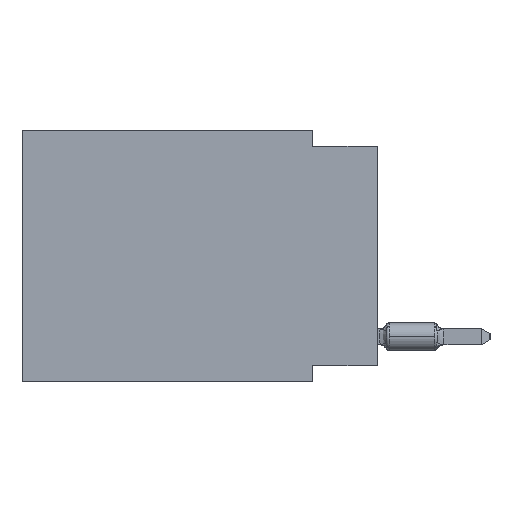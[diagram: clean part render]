
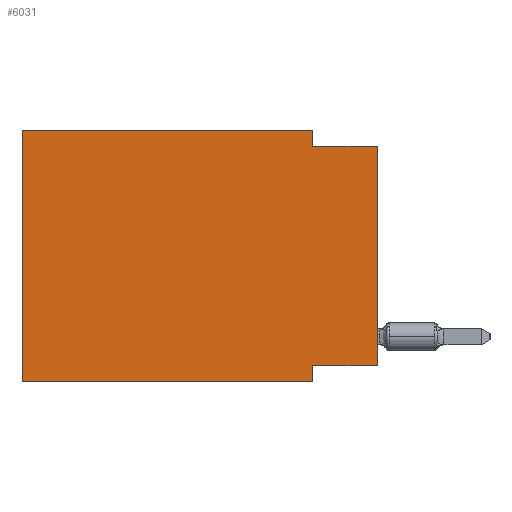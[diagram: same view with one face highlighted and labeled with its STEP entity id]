
A CAD part, left-side view. The second image highlights one B-rep face of the part: STEP entity #6031.
In plain terms, the highlighted planar face has unit normal (-1, 0, 0).
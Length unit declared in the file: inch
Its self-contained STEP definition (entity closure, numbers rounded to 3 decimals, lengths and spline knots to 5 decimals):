
#809 = CARTESIAN_POINT ( 'NONE',  ( 0., 0.55, 0. ) ) ;
#1346 = DIRECTION ( 'NONE',  ( 0., -1., 0. ) ) ;
#1994 = VERTEX_POINT ( 'NONE', #16674 ) ;
#2428 = VECTOR ( 'NONE', #15938, 39.37008 ) ;
#3640 = CARTESIAN_POINT ( 'NONE',  ( 0., 0.55, 0. ) ) ;
#3783 = VERTEX_POINT ( 'NONE', #4040 ) ;
#3809 = CARTESIAN_POINT ( 'NONE',  ( 0., 0.1, -0.39 ) ) ;
#4040 = CARTESIAN_POINT ( 'NONE',  ( 0., 0., -0.365 ) ) ;
#4198 = CARTESIAN_POINT ( 'NONE',  ( 0., 0.55, -0.39 ) ) ;
#4625 = LINE ( 'NONE', #8189, #2428 ) ;
#5137 = CARTESIAN_POINT ( 'NONE',  ( 0., 0.1, 0. ) ) ;
#5766 = VECTOR ( 'NONE', #21527, 39.37008 ) ;
#6031 = ADVANCED_FACE ( 'NONE', ( #18862 ), #15040, .F. ) ;
#6274 = VERTEX_POINT ( 'NONE', #12842 ) ;
#7086 = LINE ( 'NONE', #3640, #7305 ) ;
#7305 = VECTOR ( 'NONE', #1346, 39.37008 ) ;
#8126 = ORIENTED_EDGE ( 'NONE', *, *, #13465, .T. ) ;
#8189 = CARTESIAN_POINT ( 'NONE',  ( 0., 0., 0. ) ) ;
#8233 = LINE ( 'NONE', #11546, #16491 ) ;
#8669 = DIRECTION ( 'NONE',  ( 0., 0., 1. ) ) ;
#8681 = EDGE_CURVE ( 'NONE', #11256, #14392, #10576, .T. ) ;
#9122 = ORIENTED_EDGE ( 'NONE', *, *, #15494, .F. ) ;
#10052 = LINE ( 'NONE', #17442, #5766 ) ;
#10292 = CARTESIAN_POINT ( 'NONE',  ( 0., 0.1, -0.025 ) ) ;
#10576 = LINE ( 'NONE', #18341, #19869 ) ;
#10843 = ORIENTED_EDGE ( 'NONE', *, *, #23751, .F. ) ;
#10985 = VERTEX_POINT ( 'NONE', #12377 ) ;
#11223 = DIRECTION ( 'NONE',  ( 1., 0., 0. ) ) ;
#11256 = VERTEX_POINT ( 'NONE', #4198 ) ;
#11487 = DIRECTION ( 'NONE',  ( 0., 0., -1. ) ) ;
#11546 = CARTESIAN_POINT ( 'NONE',  ( 0., 0., -0.025 ) ) ;
#12377 = CARTESIAN_POINT ( 'NONE',  ( 0., 0.1, -0.365 ) ) ;
#12579 = VECTOR ( 'NONE', #22831, 39.37008 ) ;
#12674 = LINE ( 'NONE', #18514, #23748 ) ;
#12842 = CARTESIAN_POINT ( 'NONE',  ( 0., 0., -0.025 ) ) ;
#13453 = DIRECTION ( 'NONE',  ( 0., -1., 0. ) ) ;
#13465 = EDGE_CURVE ( 'NONE', #11256, #23709, #10052, .T. ) ;
#13955 = EDGE_CURVE ( 'NONE', #3783, #10985, #12674, .T. ) ;
#14392 = VERTEX_POINT ( 'NONE', #809 ) ;
#14685 = ORIENTED_EDGE ( 'NONE', *, *, #8681, .F. ) ;
#14923 = DIRECTION ( 'NONE',  ( 0., 0., -1. ) ) ;
#15040 = PLANE ( 'NONE',  #18282 ) ;
#15173 = LINE ( 'NONE', #22939, #23479 ) ;
#15293 = LINE ( 'NONE', #5137, #12579 ) ;
#15321 = VERTEX_POINT ( 'NONE', #10292 ) ;
#15494 = EDGE_CURVE ( 'NONE', #15321, #6274, #8233, .T. ) ;
#15938 = DIRECTION ( 'NONE',  ( 0., 0., 1. ) ) ;
#16491 = VECTOR ( 'NONE', #13453, 39.37008 ) ;
#16674 = CARTESIAN_POINT ( 'NONE',  ( 0., 0.1, 0. ) ) ;
#17442 = CARTESIAN_POINT ( 'NONE',  ( 0., 0.55, -0.39 ) ) ;
#17772 = ORIENTED_EDGE ( 'NONE', *, *, #24307, .F. ) ;
#18282 = AXIS2_PLACEMENT_3D ( 'NONE', #19356, #11223, #11487 ) ;
#18341 = CARTESIAN_POINT ( 'NONE',  ( 0., 0.55, 0. ) ) ;
#18514 = CARTESIAN_POINT ( 'NONE',  ( 0., 0., -0.365 ) ) ;
#18644 = DIRECTION ( 'NONE',  ( 0., 1., 0. ) ) ;
#18862 = FACE_OUTER_BOUND ( 'NONE', #20756, .T. ) ;
#19356 = CARTESIAN_POINT ( 'NONE',  ( 0., 0.55, 0. ) ) ;
#19398 = ORIENTED_EDGE ( 'NONE', *, *, #13955, .F. ) ;
#19423 = ORIENTED_EDGE ( 'NONE', *, *, #19471, .T. ) ;
#19471 = EDGE_CURVE ( 'NONE', #3783, #6274, #4625, .T. ) ;
#19869 = VECTOR ( 'NONE', #8669, 39.37008 ) ;
#20756 = EDGE_LOOP ( 'NONE', ( #19423, #9122, #22992, #10843, #14685, #8126, #17772, #19398 ) ) ;
#21527 = DIRECTION ( 'NONE',  ( 0., -1., 0. ) ) ;
#22831 = DIRECTION ( 'NONE',  ( 0., 0., -1. ) ) ;
#22939 = CARTESIAN_POINT ( 'NONE',  ( 0., 0.1, -0.39 ) ) ;
#22992 = ORIENTED_EDGE ( 'NONE', *, *, #24275, .F. ) ;
#23479 = VECTOR ( 'NONE', #14923, 39.37008 ) ;
#23709 = VERTEX_POINT ( 'NONE', #3809 ) ;
#23748 = VECTOR ( 'NONE', #18644, 39.37008 ) ;
#23751 = EDGE_CURVE ( 'NONE', #14392, #1994, #7086, .T. ) ;
#24275 = EDGE_CURVE ( 'NONE', #1994, #15321, #15293, .T. ) ;
#24307 = EDGE_CURVE ( 'NONE', #10985, #23709, #15173, .T. ) ;
